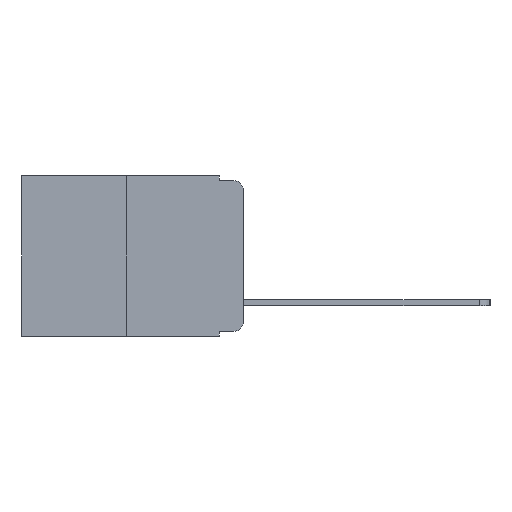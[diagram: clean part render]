
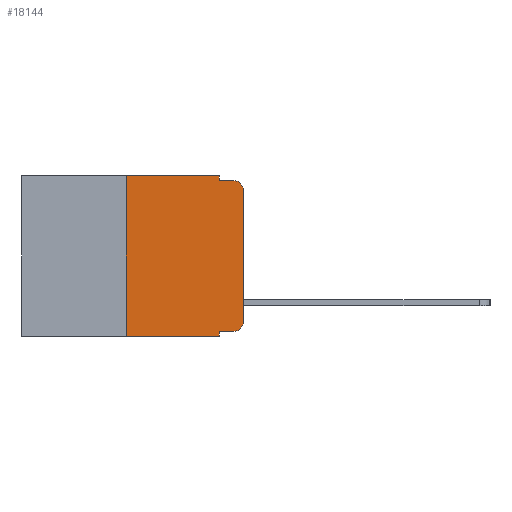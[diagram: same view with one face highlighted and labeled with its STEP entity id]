
A CAD part, left-side view. The second image highlights one B-rep face of the part: STEP entity #18144.
In plain terms, the highlighted planar face has unit normal (-1, 0, 0).
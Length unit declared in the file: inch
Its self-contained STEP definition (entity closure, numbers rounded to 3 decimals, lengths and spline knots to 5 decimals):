
#145 = VERTEX_POINT ( 'NONE', #21941 ) ;
#863 = CARTESIAN_POINT ( 'NONE',  ( 0., 0., -0.313 ) ) ;
#1504 = LINE ( 'NONE', #22898, #10449 ) ;
#1599 = EDGE_CURVE ( 'NONE', #9058, #17460, #8272, .T. ) ;
#1602 = LINE ( 'NONE', #9690, #15279 ) ;
#1664 = DIRECTION ( 'NONE',  ( 0., 0., 1. ) ) ;
#1954 = CARTESIAN_POINT ( 'NONE',  ( 0., 0.051, -0.333 ) ) ;
#2132 = CARTESIAN_POINT ( 'NONE',  ( 0., 0.051, -0.333 ) ) ;
#2663 = AXIS2_PLACEMENT_3D ( 'NONE', #14882, #4193, #16665 ) ;
#2808 = EDGE_CURVE ( 'NONE', #17460, #12690, #7140, .T. ) ;
#4011 = AXIS2_PLACEMENT_3D ( 'NONE', #20014, #9408, #21757 ) ;
#4193 = DIRECTION ( 'NONE',  ( -1., 0., 0. ) ) ;
#4409 = CARTESIAN_POINT ( 'NONE',  ( 0., 0.02, -0.01 ) ) ;
#4420 = ORIENTED_EDGE ( 'NONE', *, *, #16402, .T. ) ;
#4512 = ORIENTED_EDGE ( 'NONE', *, *, #17598, .T. ) ;
#4605 = VERTEX_POINT ( 'NONE', #14329 ) ;
#4607 = ORIENTED_EDGE ( 'NONE', *, *, #18766, .F. ) ;
#4933 = ORIENTED_EDGE ( 'NONE', *, *, #20240, .T. ) ;
#5002 = ORIENTED_EDGE ( 'NONE', *, *, #22272, .F. ) ;
#5051 = ORIENTED_EDGE ( 'NONE', *, *, #10599, .F. ) ;
#5128 = AXIS2_PLACEMENT_3D ( 'NONE', #5623, #21577, #10994 ) ;
#5222 = EDGE_CURVE ( 'NONE', #20518, #12690, #7915, .T. ) ;
#5337 = LINE ( 'NONE', #21562, #18948 ) ;
#5365 = VERTEX_POINT ( 'NONE', #863 ) ;
#5623 = CARTESIAN_POINT ( 'NONE',  ( 0., 0.473, 0. ) ) ;
#5701 = VERTEX_POINT ( 'NONE', #1954 ) ;
#5828 = ORIENTED_EDGE ( 'NONE', *, *, #1599, .F. ) ;
#5927 = ORIENTED_EDGE ( 'NONE', *, *, #2808, .F. ) ;
#6393 = EDGE_CURVE ( 'NONE', #5365, #20518, #5337, .T. ) ;
#6412 = ORIENTED_EDGE ( 'NONE', *, *, #5222, .T. ) ;
#6433 = ORIENTED_EDGE ( 'NONE', *, *, #6393, .T. ) ;
#6654 = DIRECTION ( 'NONE',  ( 0., 0., -1. ) ) ;
#7140 = LINE ( 'NONE', #10103, #16019 ) ;
#7915 = CIRCLE ( 'NONE', #4011, 0.02 ) ;
#8049 = CARTESIAN_POINT ( 'NONE',  ( 0., 0.473, 0. ) ) ;
#8272 = LINE ( 'NONE', #22566, #16602 ) ;
#8525 = CIRCLE ( 'NONE', #2663, 0.02 ) ;
#9058 = VERTEX_POINT ( 'NONE', #21246 ) ;
#9219 = PLANE ( 'NONE',  #5128 ) ;
#9325 = DIRECTION ( 'NONE',  ( 0., -1., 0. ) ) ;
#9408 = DIRECTION ( 'NONE',  ( -1., 0., 0. ) ) ;
#9690 = CARTESIAN_POINT ( 'NONE',  ( 0., 0.473, -0.343 ) ) ;
#10103 = CARTESIAN_POINT ( 'NONE',  ( 0., 0.051, -0.01 ) ) ;
#10449 = VECTOR ( 'NONE', #1664, 39.37008 ) ;
#10599 = EDGE_CURVE ( 'NONE', #12437, #9058, #16960, .T. ) ;
#10630 = CARTESIAN_POINT ( 'NONE',  ( 0., 0.051, -0.01 ) ) ;
#10994 = DIRECTION ( 'NONE',  ( 0., 0., -1. ) ) ;
#11827 = LINE ( 'NONE', #2132, #15968 ) ;
#12113 = CARTESIAN_POINT ( 'NONE',  ( 0., 0., -0.03 ) ) ;
#12437 = VERTEX_POINT ( 'NONE', #16730 ) ;
#12690 = VERTEX_POINT ( 'NONE', #4409 ) ;
#13996 = CARTESIAN_POINT ( 'NONE',  ( 0., 0.25, -0.343 ) ) ;
#14329 = CARTESIAN_POINT ( 'NONE',  ( 0., 0.02, -0.333 ) ) ;
#14555 = DIRECTION ( 'NONE',  ( 0., 0., 1. ) ) ;
#14882 = CARTESIAN_POINT ( 'NONE',  ( 0., 0.02, -0.313 ) ) ;
#15279 = VECTOR ( 'NONE', #20295, 39.37008 ) ;
#15968 = VECTOR ( 'NONE', #9325, 39.37008 ) ;
#16019 = VECTOR ( 'NONE', #17182, 39.37008 ) ;
#16046 = CARTESIAN_POINT ( 'NONE',  ( 0., 0.051, 0. ) ) ;
#16402 = EDGE_CURVE ( 'NONE', #4605, #5365, #8525, .T. ) ;
#16602 = VECTOR ( 'NONE', #6654, 39.37008 ) ;
#16665 = DIRECTION ( 'NONE',  ( 0., 0., -1. ) ) ;
#16730 = CARTESIAN_POINT ( 'NONE',  ( 0., 0.25, 0. ) ) ;
#16960 = LINE ( 'NONE', #8049, #19992 ) ;
#17182 = DIRECTION ( 'NONE',  ( 0., -1., 0. ) ) ;
#17373 = VERTEX_POINT ( 'NONE', #13996 ) ;
#17460 = VERTEX_POINT ( 'NONE', #10630 ) ;
#17598 = EDGE_CURVE ( 'NONE', #5701, #4605, #11827, .T. ) ;
#18144 = ADVANCED_FACE ( 'NONE', ( #22516 ), #9219, .F. ) ;
#18677 = DIRECTION ( 'NONE',  ( 0., -1., 0. ) ) ;
#18688 = VECTOR ( 'NONE', #19532, 39.37008 ) ;
#18766 = EDGE_CURVE ( 'NONE', #5701, #145, #19239, .T. ) ;
#18948 = VECTOR ( 'NONE', #14555, 39.37008 ) ;
#19239 = LINE ( 'NONE', #16046, #18688 ) ;
#19532 = DIRECTION ( 'NONE',  ( 0., 0., -1. ) ) ;
#19992 = VECTOR ( 'NONE', #18677, 39.37008 ) ;
#20014 = CARTESIAN_POINT ( 'NONE',  ( 0., 0.02, -0.03 ) ) ;
#20240 = EDGE_CURVE ( 'NONE', #17373, #145, #1602, .T. ) ;
#20295 = DIRECTION ( 'NONE',  ( 0., -1., 0. ) ) ;
#20518 = VERTEX_POINT ( 'NONE', #12113 ) ;
#21110 = EDGE_LOOP ( 'NONE', ( #6433, #6412, #5927, #5828, #5051, #5002, #4933, #4607, #4512, #4420 ) ) ;
#21246 = CARTESIAN_POINT ( 'NONE',  ( 0., 0.051, 0. ) ) ;
#21562 = CARTESIAN_POINT ( 'NONE',  ( 0., 0., 0. ) ) ;
#21577 = DIRECTION ( 'NONE',  ( 1., 0., 0. ) ) ;
#21757 = DIRECTION ( 'NONE',  ( 0., 0., -1. ) ) ;
#21941 = CARTESIAN_POINT ( 'NONE',  ( 0., 0.051, -0.343 ) ) ;
#22272 = EDGE_CURVE ( 'NONE', #17373, #12437, #1504, .T. ) ;
#22516 = FACE_OUTER_BOUND ( 'NONE', #21110, .T. ) ;
#22566 = CARTESIAN_POINT ( 'NONE',  ( 0., 0.051, 0. ) ) ;
#22898 = CARTESIAN_POINT ( 'NONE',  ( 0., 0.25, 0. ) ) ;
